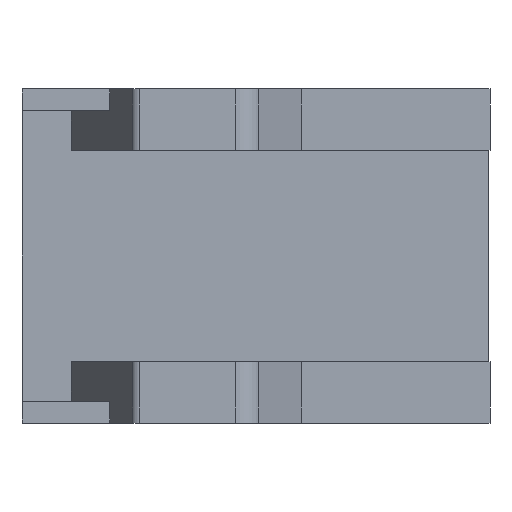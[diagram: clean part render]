
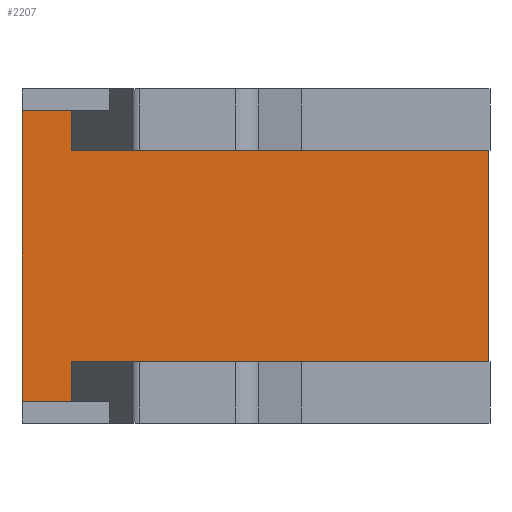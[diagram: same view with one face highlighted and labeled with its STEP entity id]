
A CAD part, left-side view. The second image highlights one B-rep face of the part: STEP entity #2207.
In plain terms, the highlighted planar face has unit normal (-1, 0, 0).
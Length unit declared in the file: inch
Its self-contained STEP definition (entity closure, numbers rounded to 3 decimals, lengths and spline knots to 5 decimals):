
#234=FACE_OUTER_BOUND('',#368,.T.);
#368=EDGE_LOOP('',(#1918,#1919,#1920,#1921,#1922,#1923,#1924,#1925));
#423=LINE('',#2967,#671);
#569=LINE('',#3586,#817);
#604=LINE('',#4017,#852);
#606=LINE('',#4022,#854);
#610=LINE('',#4030,#858);
#614=LINE('',#4044,#862);
#615=LINE('',#4045,#863);
#616=LINE('',#4046,#864);
#671=VECTOR('',#2426,0.3937);
#817=VECTOR('',#2698,0.3937);
#852=VECTOR('',#2801,0.3937);
#854=VECTOR('',#2805,0.3937);
#858=VECTOR('',#2813,0.3937);
#862=VECTOR('',#2825,0.3937);
#863=VECTOR('',#2826,0.3937);
#864=VECTOR('',#2827,0.3937);
#903=VERTEX_POINT('',#2944);
#914=VERTEX_POINT('',#2965);
#1036=VERTEX_POINT('',#3583);
#1037=VERTEX_POINT('',#3585);
#1058=VERTEX_POINT('',#4015);
#1060=VERTEX_POINT('',#4021);
#1061=VERTEX_POINT('',#4027);
#1068=VERTEX_POINT('',#4043);
#1109=EDGE_CURVE('',#914,#903,#423,.T.);
#1294=EDGE_CURVE('',#1036,#1037,#569,.T.);
#1349=EDGE_CURVE('',#914,#1058,#604,.T.);
#1351=EDGE_CURVE('',#1060,#903,#606,.T.);
#1355=EDGE_CURVE('',#1061,#1036,#610,.T.);
#1362=EDGE_CURVE('',#1068,#1037,#614,.T.);
#1363=EDGE_CURVE('',#1061,#1060,#615,.T.);
#1364=EDGE_CURVE('',#1058,#1068,#616,.T.);
#1918=ORIENTED_EDGE('',*,*,#1362,.T.);
#1919=ORIENTED_EDGE('',*,*,#1294,.F.);
#1920=ORIENTED_EDGE('',*,*,#1355,.F.);
#1921=ORIENTED_EDGE('',*,*,#1363,.T.);
#1922=ORIENTED_EDGE('',*,*,#1351,.T.);
#1923=ORIENTED_EDGE('',*,*,#1109,.F.);
#1924=ORIENTED_EDGE('',*,*,#1349,.T.);
#1925=ORIENTED_EDGE('',*,*,#1364,.T.);
#2090=PLANE('',#2353);
#2207=ADVANCED_FACE('',(#234),#2090,.F.);
#2353=AXIS2_PLACEMENT_3D('',#4042,#2823,#2824);
#2426=DIRECTION('',(0.,0.,1.));
#2698=DIRECTION('',(0.,0.,-1.));
#2801=DIRECTION('',(0.,-1.,0.));
#2805=DIRECTION('',(0.,1.,0.));
#2813=DIRECTION('',(0.,-1.,0.));
#2823=DIRECTION('center_axis',(1.,0.,0.));
#2824=DIRECTION('ref_axis',(0.,0.,1.));
#2825=DIRECTION('',(0.,-1.,0.));
#2826=DIRECTION('',(0.,0.,1.));
#2827=DIRECTION('',(0.,0.,1.));
#2944=CARTESIAN_POINT('',(0.4893,2.0945,1.39765));
#2965=CARTESIAN_POINT('',(0.4893,2.0945,0.09845));
#2967=CARTESIAN_POINT('',(0.4893,2.0945,0.37403));
#3583=CARTESIAN_POINT('',(0.4893,0.00861,1.2205));
#3585=CARTESIAN_POINT('',(0.4893,0.00861,0.2756));
#3586=CARTESIAN_POINT('',(0.4893,0.00861,0.1378));
#4015=CARTESIAN_POINT('',(0.4893,1.87332,0.09845));
#4017=CARTESIAN_POINT('',(0.4893,1.87332,0.09845));
#4021=CARTESIAN_POINT('',(0.4893,1.87332,1.39765));
#4022=CARTESIAN_POINT('',(0.4893,1.87332,1.39765));
#4027=CARTESIAN_POINT('',(0.4893,1.87332,1.2205));
#4030=CARTESIAN_POINT('',(0.4893,2.0945,1.2205));
#4042=CARTESIAN_POINT('Origin',(0.4893,2.0945,0.2756));
#4043=CARTESIAN_POINT('',(0.4893,1.87332,0.2756));
#4044=CARTESIAN_POINT('',(0.4893,2.0945,0.2756));
#4045=CARTESIAN_POINT('',(0.4893,1.87332,0.74805));
#4046=CARTESIAN_POINT('',(0.4893,1.87332,0.74805));
